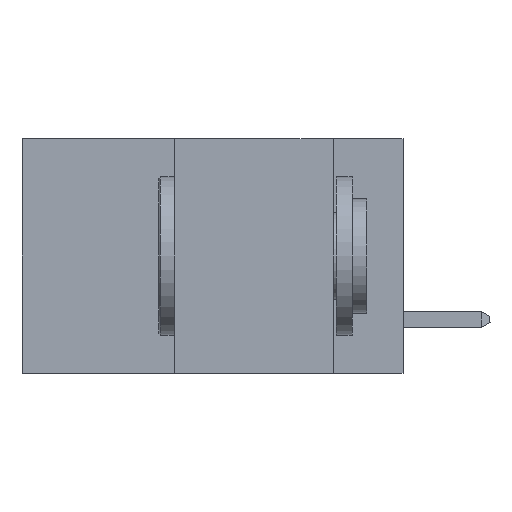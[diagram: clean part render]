
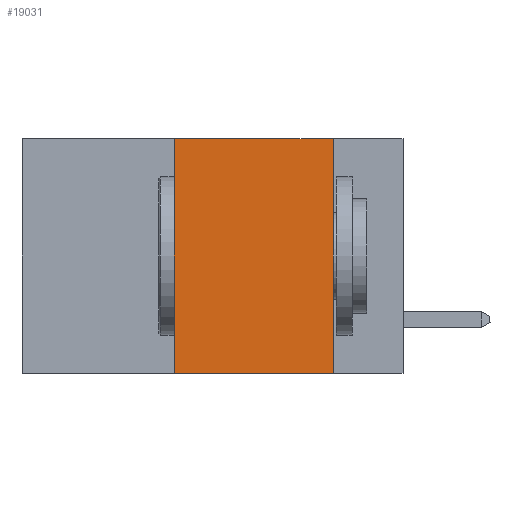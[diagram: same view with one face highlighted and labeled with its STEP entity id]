
A CAD part, left-side view. The second image highlights one B-rep face of the part: STEP entity #19031.
In plain terms, the highlighted planar face has unit normal (-1, 0, 0).
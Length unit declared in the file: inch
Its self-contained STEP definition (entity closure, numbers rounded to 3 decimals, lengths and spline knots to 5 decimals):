
#654 = ORIENTED_EDGE ( 'NONE', *, *, #17053, .F. ) ;
#1743 = VERTEX_POINT ( 'NONE', #16328 ) ;
#2839 = DIRECTION ( 'NONE',  ( 1., 0., 0. ) ) ;
#3408 = ORIENTED_EDGE ( 'NONE', *, *, #14512, .F. ) ;
#4001 = LINE ( 'NONE', #11460, #25855 ) ;
#4162 = CARTESIAN_POINT ( 'NONE',  ( 0., 0.36, 0. ) ) ;
#4417 = DIRECTION ( 'NONE',  ( 0., -1., 0. ) ) ;
#5941 = DIRECTION ( 'NONE',  ( 0., 0., -1. ) ) ;
#7124 = ORIENTED_EDGE ( 'NONE', *, *, #31481, .T. ) ;
#8007 = CARTESIAN_POINT ( 'NONE',  ( 0., 0.11, 0. ) ) ;
#9313 = DIRECTION ( 'NONE',  ( 0., -1., 0. ) ) ;
#10272 = VERTEX_POINT ( 'NONE', #12988 ) ;
#11460 = CARTESIAN_POINT ( 'NONE',  ( 0., 0.11, 0. ) ) ;
#11928 = ORIENTED_EDGE ( 'NONE', *, *, #32859, .F. ) ;
#12521 = CARTESIAN_POINT ( 'NONE',  ( 0., 0.36, -0.37 ) ) ;
#12696 = VERTEX_POINT ( 'NONE', #8007 ) ;
#12988 = CARTESIAN_POINT ( 'NONE',  ( 0., 0.36, 0. ) ) ;
#14512 = EDGE_CURVE ( 'NONE', #28839, #10272, #24030, .T. ) ;
#14836 = DIRECTION ( 'NONE',  ( 0., 0., 1. ) ) ;
#16328 = CARTESIAN_POINT ( 'NONE',  ( 0., 0.11, -0.37 ) ) ;
#17053 = EDGE_CURVE ( 'NONE', #12696, #1743, #4001, .T. ) ;
#18426 = LINE ( 'NONE', #31212, #34310 ) ;
#19031 = ADVANCED_FACE ( 'NONE', ( #30065 ), #21527, .F. ) ;
#21527 = PLANE ( 'NONE',  #23838 ) ;
#22193 = VECTOR ( 'NONE', #4417, 39.37008 ) ;
#22307 = VECTOR ( 'NONE', #14836, 39.37008 ) ;
#23440 = CARTESIAN_POINT ( 'NONE',  ( 0., 0.6, 0. ) ) ;
#23838 = AXIS2_PLACEMENT_3D ( 'NONE', #30274, #2839, #32932 ) ;
#24030 = LINE ( 'NONE', #4162, #22307 ) ;
#24332 = LINE ( 'NONE', #23440, #22193 ) ;
#25855 = VECTOR ( 'NONE', #5941, 39.37008 ) ;
#28839 = VERTEX_POINT ( 'NONE', #12521 ) ;
#30065 = FACE_OUTER_BOUND ( 'NONE', #32573, .T. ) ;
#30274 = CARTESIAN_POINT ( 'NONE',  ( 0., 0.6, 0. ) ) ;
#31212 = CARTESIAN_POINT ( 'NONE',  ( 0., 0.6, -0.37 ) ) ;
#31481 = EDGE_CURVE ( 'NONE', #28839, #1743, #18426, .T. ) ;
#32573 = EDGE_LOOP ( 'NONE', ( #654, #11928, #3408, #7124 ) ) ;
#32859 = EDGE_CURVE ( 'NONE', #10272, #12696, #24332, .T. ) ;
#32932 = DIRECTION ( 'NONE',  ( 0., 0., -1. ) ) ;
#34310 = VECTOR ( 'NONE', #9313, 39.37008 ) ;
